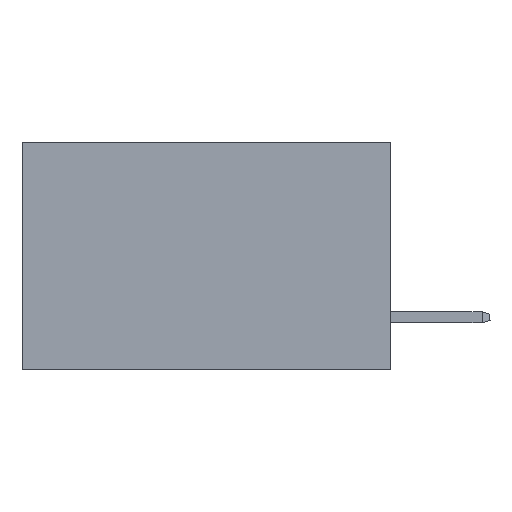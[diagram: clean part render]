
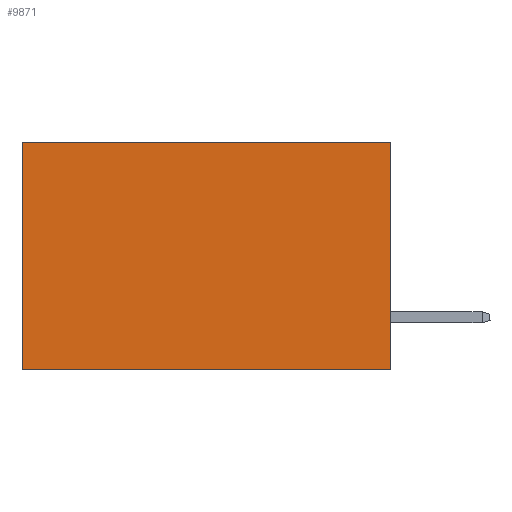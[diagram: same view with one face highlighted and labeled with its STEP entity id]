
A CAD part, left-side view. The second image highlights one B-rep face of the part: STEP entity #9871.
In plain terms, the highlighted planar face has unit normal (-1, 0, 0).
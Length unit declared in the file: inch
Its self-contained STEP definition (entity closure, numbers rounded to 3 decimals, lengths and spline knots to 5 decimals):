
#529 = DIRECTION ( 'NONE',  ( 1., 0., 0. ) ) ;
#2276 = ORIENTED_EDGE ( 'NONE', *, *, #9580, .F. ) ;
#3006 = ORIENTED_EDGE ( 'NONE', *, *, #12932, .T. ) ;
#3117 = LINE ( 'NONE', #23310, #6540 ) ;
#3562 = VECTOR ( 'NONE', #7887, 39.37008 ) ;
#3604 = EDGE_CURVE ( 'NONE', #5856, #18226, #3117, .T. ) ;
#4400 = FACE_OUTER_BOUND ( 'NONE', #18074, .T. ) ;
#4758 = PLANE ( 'NONE',  #18297 ) ;
#5856 = VERTEX_POINT ( 'NONE', #18756 ) ;
#6540 = VECTOR ( 'NONE', #12569, 39.37008 ) ;
#6693 = VECTOR ( 'NONE', #14175, 39.37008 ) ;
#6976 = VERTEX_POINT ( 'NONE', #13124 ) ;
#7743 = VECTOR ( 'NONE', #20995, 39.37008 ) ;
#7887 = DIRECTION ( 'NONE',  ( 0., 1., 0. ) ) ;
#9580 = EDGE_CURVE ( 'NONE', #12166, #18226, #16361, .T. ) ;
#9871 = ADVANCED_FACE ( 'NONE', ( #4400 ), #4758, .F. ) ;
#10123 = CARTESIAN_POINT ( 'NONE',  ( 0.2875, 0., -0.37 ) ) ;
#11230 = EDGE_CURVE ( 'NONE', #6976, #12166, #22632, .T. ) ;
#11485 = CARTESIAN_POINT ( 'NONE',  ( 0.2875, 0., -0.37 ) ) ;
#11553 = CARTESIAN_POINT ( 'NONE',  ( 0.2875, 0., 0. ) ) ;
#12166 = VERTEX_POINT ( 'NONE', #10123 ) ;
#12569 = DIRECTION ( 'NONE',  ( 0., 0., -1. ) ) ;
#12932 = EDGE_CURVE ( 'NONE', #6976, #5856, #14479, .T. ) ;
#13124 = CARTESIAN_POINT ( 'NONE',  ( 0.2875, 0., 0. ) ) ;
#14175 = DIRECTION ( 'NONE',  ( 0., 0., -1. ) ) ;
#14479 = LINE ( 'NONE', #17837, #7743 ) ;
#14498 = ORIENTED_EDGE ( 'NONE', *, *, #3604, .T. ) ;
#15054 = CARTESIAN_POINT ( 'NONE',  ( 0.2875, 0.6, -0.37 ) ) ;
#16361 = LINE ( 'NONE', #11485, #3562 ) ;
#17837 = CARTESIAN_POINT ( 'NONE',  ( 0.2875, 0., 0. ) ) ;
#18074 = EDGE_LOOP ( 'NONE', ( #14498, #2276, #23845, #3006 ) ) ;
#18226 = VERTEX_POINT ( 'NONE', #15054 ) ;
#18297 = AXIS2_PLACEMENT_3D ( 'NONE', #18872, #529, #21127 ) ;
#18756 = CARTESIAN_POINT ( 'NONE',  ( 0.2875, 0.6, 0. ) ) ;
#18872 = CARTESIAN_POINT ( 'NONE',  ( 0.2875, 0., 0. ) ) ;
#20995 = DIRECTION ( 'NONE',  ( 0., 1., 0. ) ) ;
#21127 = DIRECTION ( 'NONE',  ( 0., 0., -1. ) ) ;
#22632 = LINE ( 'NONE', #11553, #6693 ) ;
#23310 = CARTESIAN_POINT ( 'NONE',  ( 0.2875, 0.6, 0. ) ) ;
#23845 = ORIENTED_EDGE ( 'NONE', *, *, #11230, .F. ) ;
